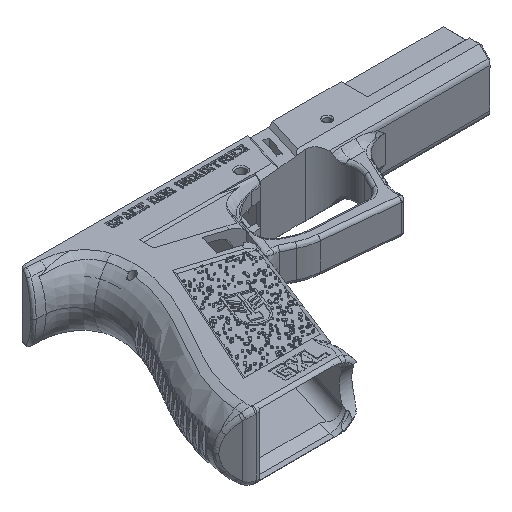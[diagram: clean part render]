
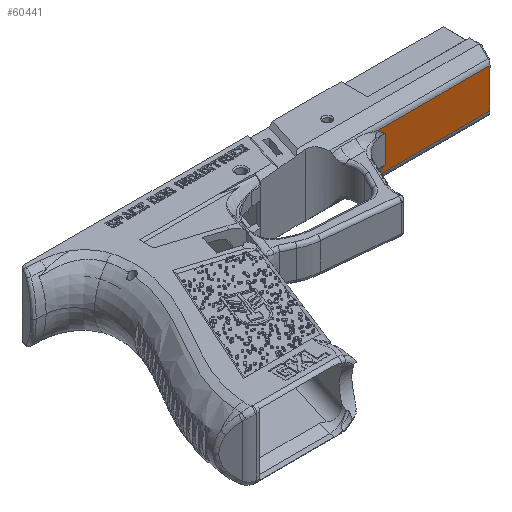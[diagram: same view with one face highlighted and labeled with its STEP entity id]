
A CAD part, isometric view. The second image highlights one B-rep face of the part: STEP entity #60441.
In plain terms, the highlighted planar face has unit normal (0, -1, 0).
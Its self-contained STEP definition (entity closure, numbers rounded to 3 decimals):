
#6654=B_SPLINE_CURVE_WITH_KNOTS('',3,(#85369,#85370,#85371,#85372,#85373,
#85374),.UNSPECIFIED.,.F.,.F.,(4,2,4),(-0.427,0.,0.001),
 .UNSPECIFIED.);
#7289=B_SPLINE_CURVE_WITH_KNOTS('',3,(#111242,#111243,#111244,#111245,#111246,
#111247),.UNSPECIFIED.,.F.,.F.,(4,2,4),(-1.495,-1.493,
-1.066),.UNSPECIFIED.);
#10037=FACE_OUTER_BOUND('',#13810,.T.);
#13810=EDGE_LOOP('',(#48246,#48247,#48248,#48249,#48250,#48251));
#17651=LINE('',#106208,#21495);
#17770=LINE('',#111231,#21614);
#17771=LINE('',#111239,#21615);
#17772=LINE('',#111241,#21616);
#21495=VECTOR('',#66609,3.);
#21614=VECTOR('',#66912,10.);
#21615=VECTOR('',#66915,10.);
#21616=VECTOR('',#66916,3.);
#24347=VERTEX_POINT('',#85144);
#24353=VERTEX_POINT('',#85337);
#26492=VERTEX_POINT('',#106203);
#27131=VERTEX_POINT('',#111230);
#27132=VERTEX_POINT('',#111238);
#27133=VERTEX_POINT('',#111240);
#30721=EDGE_CURVE('',#24353,#24347,#6654,.T.);
#34011=EDGE_CURVE('',#26492,#24353,#17651,.T.);
#34759=EDGE_CURVE('',#24347,#27131,#17770,.T.);
#34761=EDGE_CURVE('',#27132,#26492,#17771,.T.);
#34762=EDGE_CURVE('',#27133,#27132,#17772,.T.);
#34763=EDGE_CURVE('',#27131,#27133,#7289,.T.);
#48246=ORIENTED_EDGE('',*,*,#34761,.F.);
#48247=ORIENTED_EDGE('',*,*,#34762,.F.);
#48248=ORIENTED_EDGE('',*,*,#34763,.F.);
#48249=ORIENTED_EDGE('',*,*,#34759,.F.);
#48250=ORIENTED_EDGE('',*,*,#30721,.F.);
#48251=ORIENTED_EDGE('',*,*,#34011,.F.);
#58198=PLANE('',#63013);
#60441=ADVANCED_FACE('',(#10037),#58198,.F.);
#63013=AXIS2_PLACEMENT_3D('',#111237,#66913,#66914);
#66609=DIRECTION('',(-1.,0.,0.));
#66912=DIRECTION('',(0.,0.,1.));
#66913=DIRECTION('center_axis',(0.,1.,0.));
#66914=DIRECTION('ref_axis',(0.,0.,
1.));
#66915=DIRECTION('',(0.,0.,-1.));
#66916=DIRECTION('',(1.,0.,0.));
#85144=CARTESIAN_POINT('',(111.379,-18.787,-27.432));
#85337=CARTESIAN_POINT('',(107.968,-18.787,-30.094));
#85369=CARTESIAN_POINT('Ctrl Pts',(107.968,-18.787,-30.094));
#85370=CARTESIAN_POINT('Ctrl Pts',(109.135,-18.787,-29.248));
#85371=CARTESIAN_POINT('Ctrl Pts',(110.26,-18.787,-28.337));
#85372=CARTESIAN_POINT('Ctrl Pts',(111.372,-18.787,-27.437));
#85373=CARTESIAN_POINT('Ctrl Pts',(111.375,-18.787,-27.434));
#85374=CARTESIAN_POINT('Ctrl Pts',(111.379,-18.787,-27.432));
#106203=CARTESIAN_POINT('',(157.385,-18.787,-30.094));
#106208=CARTESIAN_POINT('',(82.772,-18.787,-30.094));
#111230=CARTESIAN_POINT('',(111.379,-18.787,-15.51));
#111231=CARTESIAN_POINT('',(111.379,-18.787,-25.226));
#111237=CARTESIAN_POINT('Origin',(75.926,-18.787,-21.471));
#111238=CARTESIAN_POINT('',(157.385,-18.787,-12.847));
#111239=CARTESIAN_POINT('',(157.385,-18.787,-21.471));
#111240=CARTESIAN_POINT('',(107.968,-18.787,-12.847));
#111241=CARTESIAN_POINT('',(50.545,-18.787,-12.847));
#111242=CARTESIAN_POINT('Ctrl Pts',(111.379,-18.787,
-15.51));
#111243=CARTESIAN_POINT('Ctrl Pts',(111.375,-18.787,
-15.507));
#111244=CARTESIAN_POINT('Ctrl Pts',(111.372,-18.787,
-15.504));
#111245=CARTESIAN_POINT('Ctrl Pts',(110.26,-18.787,
-14.605));
#111246=CARTESIAN_POINT('Ctrl Pts',(109.135,-18.787,
-13.694));
#111247=CARTESIAN_POINT('Ctrl Pts',(107.968,-18.787,
-12.847));
